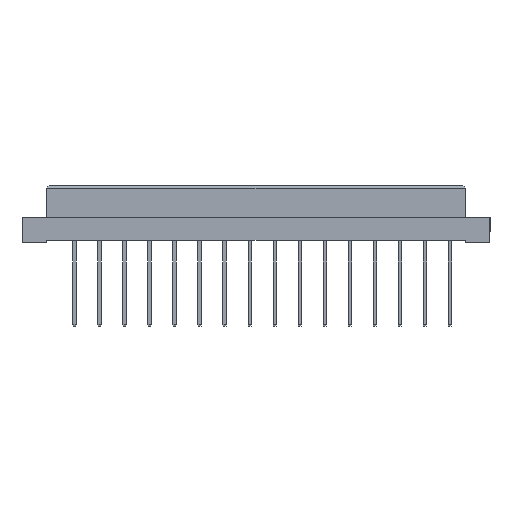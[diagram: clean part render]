
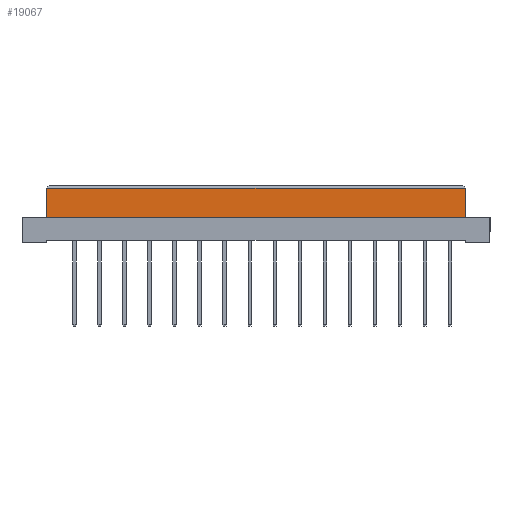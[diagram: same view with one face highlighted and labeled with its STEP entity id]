
A CAD part, top view. The second image highlights one B-rep face of the part: STEP entity #19067.
In plain terms, the highlighted planar face has unit normal (0, 0, 1).
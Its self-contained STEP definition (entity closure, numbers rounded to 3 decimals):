
#264 = LINE ( 'NONE', #29648, #19770 ) ;
#1059 = DIRECTION ( 'NONE',  ( 1., 0., 0. ) ) ;
#1450 = CARTESIAN_POINT ( 'NONE',  ( 42.5, -6.4, 4.25 ) ) ;
#3254 = CARTESIAN_POINT ( 'NONE',  ( 42.5, -6.4, 4.25 ) ) ;
#4566 = EDGE_CURVE ( 'NONE', #23300, #16118, #13547, .T. ) ;
#4902 = EDGE_LOOP ( 'NONE', ( #8693, #26234, #6411, #17490 ) ) ;
#5520 = VERTEX_POINT ( 'NONE', #20220 ) ;
#5946 = DIRECTION ( 'NONE',  ( 1., 0., 0. ) ) ;
#6411 = ORIENTED_EDGE ( 'NONE', *, *, #27891, .F. ) ;
#6627 = VERTEX_POINT ( 'NONE', #13848 ) ;
#6666 = CARTESIAN_POINT ( 'NONE',  ( 42.5, -0.5, 4.25 ) ) ;
#8047 = CARTESIAN_POINT ( 'NONE',  ( 42.5, -6.4, 4.25 ) ) ;
#8693 = ORIENTED_EDGE ( 'NONE', *, *, #19307, .T. ) ;
#11206 = VECTOR ( 'NONE', #1059, 1000. ) ;
#13048 = LINE ( 'NONE', #1450, #11206 ) ;
#13547 = LINE ( 'NONE', #22249, #23437 ) ;
#13848 = CARTESIAN_POINT ( 'NONE',  ( -42.5, -6.4, 4.25 ) ) ;
#14874 = CARTESIAN_POINT ( 'NONE',  ( -42.5, -0.5, 4.25 ) ) ;
#16118 = VERTEX_POINT ( 'NONE', #14874 ) ;
#16647 = DIRECTION ( 'NONE',  ( -1., 0., 0. ) ) ;
#16945 = DIRECTION ( 'NONE',  ( 0., 1., 0. ) ) ;
#17490 = ORIENTED_EDGE ( 'NONE', *, *, #30587, .T. ) ;
#17730 = PLANE ( 'NONE',  #31484 ) ;
#19067 = ADVANCED_FACE ( 'NONE', ( #26455 ), #17730, .T. ) ;
#19138 = VECTOR ( 'NONE', #16945, 1000. ) ;
#19307 = EDGE_CURVE ( 'NONE', #5520, #23300, #25648, .T. ) ;
#19770 = VECTOR ( 'NONE', #23086, 1000. ) ;
#20220 = CARTESIAN_POINT ( 'NONE',  ( 42.5, -6.4, 4.25 ) ) ;
#22249 = CARTESIAN_POINT ( 'NONE',  ( -42.5, -0.5, 4.25 ) ) ;
#23086 = DIRECTION ( 'NONE',  ( 0., 1., 0. ) ) ;
#23300 = VERTEX_POINT ( 'NONE', #6666 ) ;
#23437 = VECTOR ( 'NONE', #16647, 1000. ) ;
#25648 = LINE ( 'NONE', #8047, #19138 ) ;
#26234 = ORIENTED_EDGE ( 'NONE', *, *, #4566, .T. ) ;
#26455 = FACE_OUTER_BOUND ( 'NONE', #4902, .T. ) ;
#27891 = EDGE_CURVE ( 'NONE', #6627, #16118, #264, .T. ) ;
#29648 = CARTESIAN_POINT ( 'NONE',  ( -42.5, -6.4, 4.25 ) ) ;
#30587 = EDGE_CURVE ( 'NONE', #6627, #5520, #13048, .T. ) ;
#31484 = AXIS2_PLACEMENT_3D ( 'NONE', #3254, #32608, #5946 ) ;
#32608 = DIRECTION ( 'NONE',  ( 0., 0., 1. ) ) ;
